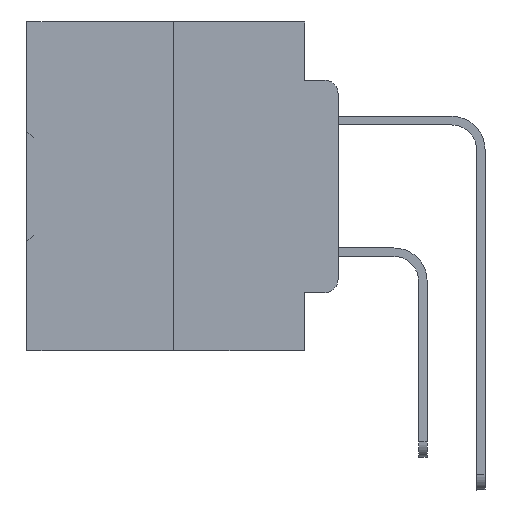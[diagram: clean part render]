
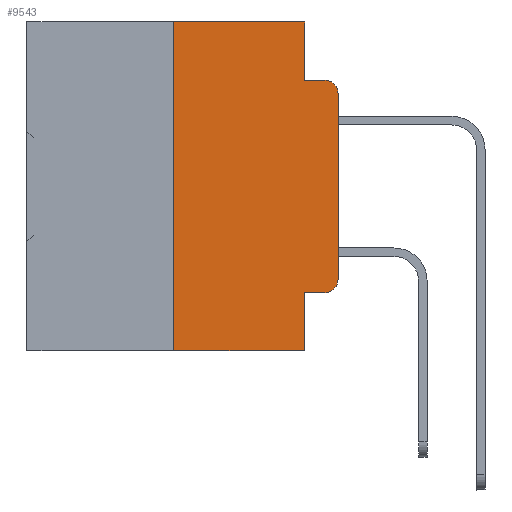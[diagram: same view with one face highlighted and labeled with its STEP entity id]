
A CAD part, left-side view. The second image highlights one B-rep face of the part: STEP entity #9543.
In plain terms, the highlighted planar face has unit normal (-1, 0, 0).
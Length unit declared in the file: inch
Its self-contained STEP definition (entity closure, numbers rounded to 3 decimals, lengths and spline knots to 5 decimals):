
#644 = EDGE_CURVE ( 'NONE', #7731, #25173, #32921, .T. ) ;
#1133 = AXIS2_PLACEMENT_3D ( 'NONE', #8205, #39374, #26603 ) ;
#1391 = LINE ( 'NONE', #13380, #24364 ) ;
#2304 = CARTESIAN_POINT ( 'NONE',  ( 0., 0.25, 0. ) ) ;
#3207 = DIRECTION ( 'NONE',  ( 1., 0., 0. ) ) ;
#3570 = EDGE_CURVE ( 'NONE', #23320, #25173, #33106, .T. ) ;
#5803 = DIRECTION ( 'NONE',  ( 0., 0., -1. ) ) ;
#6101 = DIRECTION ( 'NONE',  ( 0., -1., 0. ) ) ;
#6878 = EDGE_CURVE ( 'NONE', #23320, #7092, #31085, .T. ) ;
#7092 = VERTEX_POINT ( 'NONE', #19117 ) ;
#7404 = CARTESIAN_POINT ( 'NONE',  ( 0., 0.473, 0. ) ) ;
#7731 = VERTEX_POINT ( 'NONE', #10902 ) ;
#7870 = EDGE_CURVE ( 'NONE', #32205, #30517, #28034, .T. ) ;
#8205 = CARTESIAN_POINT ( 'NONE',  ( 0., 0.02, -0.3915 ) ) ;
#8815 = VECTOR ( 'NONE', #35195, 39.37008 ) ;
#9130 = EDGE_CURVE ( 'NONE', #39834, #29153, #28579, .T. ) ;
#9543 = ADVANCED_FACE ( 'NONE', ( #11894 ), #21825, .F. ) ;
#9677 = EDGE_CURVE ( 'NONE', #32559, #39834, #25731, .T. ) ;
#9768 = CARTESIAN_POINT ( 'NONE',  ( 0., 0.25, 0. ) ) ;
#10625 = CARTESIAN_POINT ( 'NONE',  ( 0., 0.473, -0.5 ) ) ;
#10891 = DIRECTION ( 'NONE',  ( 0., -1., 0. ) ) ;
#10902 = CARTESIAN_POINT ( 'NONE',  ( 0., 0.25, -0.5 ) ) ;
#11894 = FACE_OUTER_BOUND ( 'NONE', #12462, .T. ) ;
#12462 = EDGE_LOOP ( 'NONE', ( #15686, #39360, #16234, #16763, #25472, #33019, #35769, #13989, #39739, #21816 ) ) ;
#13380 = CARTESIAN_POINT ( 'NONE',  ( 0., 0.051, -0.0885 ) ) ;
#13989 = ORIENTED_EDGE ( 'NONE', *, *, #3570, .F. ) ;
#14354 = DIRECTION ( 'NONE',  ( 0., -1., 0. ) ) ;
#14900 = DIRECTION ( 'NONE',  ( 0., 0., 1. ) ) ;
#15686 = ORIENTED_EDGE ( 'NONE', *, *, #9677, .T. ) ;
#16234 = ORIENTED_EDGE ( 'NONE', *, *, #23482, .F. ) ;
#16523 = VECTOR ( 'NONE', #26713, 39.37008 ) ;
#16763 = ORIENTED_EDGE ( 'NONE', *, *, #7870, .F. ) ;
#17330 = LINE ( 'NONE', #7404, #25644 ) ;
#17847 = EDGE_CURVE ( 'NONE', #37605, #32205, #17330, .T. ) ;
#18061 = CARTESIAN_POINT ( 'NONE',  ( 0., 0.02, -0.0885 ) ) ;
#18199 = DIRECTION ( 'NONE',  ( -1., 0., 0. ) ) ;
#18320 = CARTESIAN_POINT ( 'NONE',  ( 0., 0.051, -0.0885 ) ) ;
#18956 = CIRCLE ( 'NONE', #1133, 0.02 ) ;
#19117 = CARTESIAN_POINT ( 'NONE',  ( 0., 0.02, -0.4115 ) ) ;
#19131 = CARTESIAN_POINT ( 'NONE',  ( 0., 0.473, 0. ) ) ;
#20283 = VECTOR ( 'NONE', #14354, 39.37008 ) ;
#21217 = CARTESIAN_POINT ( 'NONE',  ( 0., 0.051, -0.4115 ) ) ;
#21816 = ORIENTED_EDGE ( 'NONE', *, *, #26696, .T. ) ;
#21825 = PLANE ( 'NONE',  #29251 ) ;
#23320 = VERTEX_POINT ( 'NONE', #37361 ) ;
#23362 = VECTOR ( 'NONE', #6101, 39.37008 ) ;
#23476 = DIRECTION ( 'NONE',  ( 0., -1., 0. ) ) ;
#23482 = EDGE_CURVE ( 'NONE', #30517, #29153, #1391, .T. ) ;
#23831 = CARTESIAN_POINT ( 'NONE',  ( 0., 0.051, 0. ) ) ;
#23886 = VECTOR ( 'NONE', #37306, 39.37008 ) ;
#24188 = CARTESIAN_POINT ( 'NONE',  ( 0., 0.02, -0.1085 ) ) ;
#24364 = VECTOR ( 'NONE', #23476, 39.37008 ) ;
#24508 = DIRECTION ( 'NONE',  ( 0., 0., -1. ) ) ;
#24558 = CARTESIAN_POINT ( 'NONE',  ( 0., 0.051, -0.5 ) ) ;
#25173 = VERTEX_POINT ( 'NONE', #24558 ) ;
#25472 = ORIENTED_EDGE ( 'NONE', *, *, #17847, .F. ) ;
#25644 = VECTOR ( 'NONE', #10891, 39.37008 ) ;
#25731 = LINE ( 'NONE', #32311, #8815 ) ;
#26603 = DIRECTION ( 'NONE',  ( 0., 0., -1. ) ) ;
#26696 = EDGE_CURVE ( 'NONE', #7092, #32559, #18956, .T. ) ;
#26713 = DIRECTION ( 'NONE',  ( 0., 0., -1. ) ) ;
#28034 = LINE ( 'NONE', #40412, #23886 ) ;
#28579 = CIRCLE ( 'NONE', #33204, 0.02 ) ;
#29153 = VERTEX_POINT ( 'NONE', #18061 ) ;
#29251 = AXIS2_PLACEMENT_3D ( 'NONE', #19131, #3207, #24508 ) ;
#30517 = VERTEX_POINT ( 'NONE', #18320 ) ;
#31004 = EDGE_CURVE ( 'NONE', #7731, #37605, #33480, .T. ) ;
#31085 = LINE ( 'NONE', #21217, #23362 ) ;
#32205 = VERTEX_POINT ( 'NONE', #32540 ) ;
#32311 = CARTESIAN_POINT ( 'NONE',  ( 0., 0., 0. ) ) ;
#32540 = CARTESIAN_POINT ( 'NONE',  ( 0., 0.051, 0. ) ) ;
#32559 = VERTEX_POINT ( 'NONE', #40160 ) ;
#32921 = LINE ( 'NONE', #10625, #20283 ) ;
#33019 = ORIENTED_EDGE ( 'NONE', *, *, #31004, .F. ) ;
#33106 = LINE ( 'NONE', #23831, #16523 ) ;
#33204 = AXIS2_PLACEMENT_3D ( 'NONE', #24188, #18199, #5803 ) ;
#33480 = LINE ( 'NONE', #2304, #33614 ) ;
#33614 = VECTOR ( 'NONE', #14900, 39.37008 ) ;
#34840 = CARTESIAN_POINT ( 'NONE',  ( 0., 0., -0.1085 ) ) ;
#35195 = DIRECTION ( 'NONE',  ( 0., 0., 1. ) ) ;
#35769 = ORIENTED_EDGE ( 'NONE', *, *, #644, .T. ) ;
#37306 = DIRECTION ( 'NONE',  ( 0., 0., -1. ) ) ;
#37361 = CARTESIAN_POINT ( 'NONE',  ( 0., 0.051, -0.4115 ) ) ;
#37605 = VERTEX_POINT ( 'NONE', #9768 ) ;
#39360 = ORIENTED_EDGE ( 'NONE', *, *, #9130, .T. ) ;
#39374 = DIRECTION ( 'NONE',  ( -1., 0., 0. ) ) ;
#39739 = ORIENTED_EDGE ( 'NONE', *, *, #6878, .T. ) ;
#39834 = VERTEX_POINT ( 'NONE', #34840 ) ;
#40160 = CARTESIAN_POINT ( 'NONE',  ( 0., 0., -0.3915 ) ) ;
#40412 = CARTESIAN_POINT ( 'NONE',  ( 0., 0.051, 0. ) ) ;
